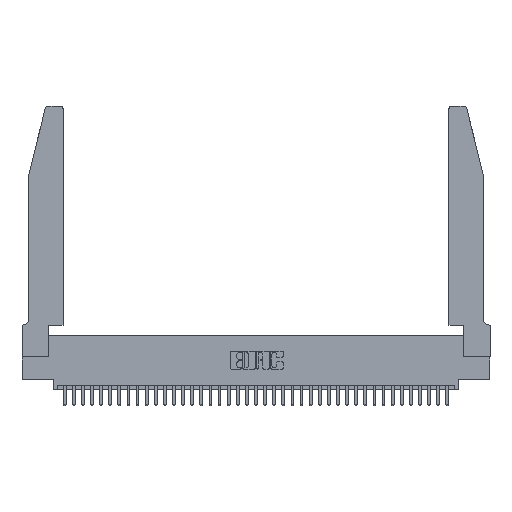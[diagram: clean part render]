
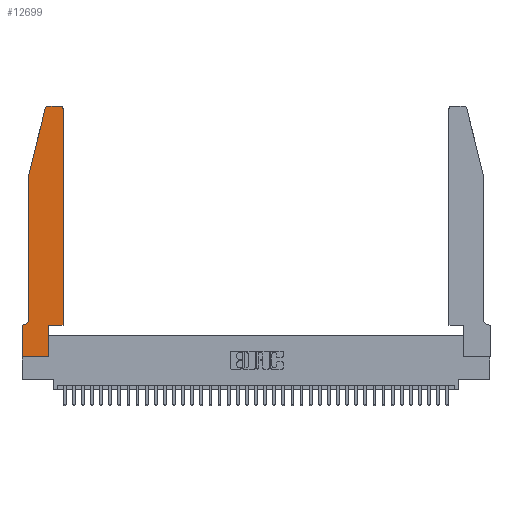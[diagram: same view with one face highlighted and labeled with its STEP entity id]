
A CAD part, top view. The second image highlights one B-rep face of the part: STEP entity #12699.
In plain terms, the highlighted planar face has unit normal (0, 0, 1).
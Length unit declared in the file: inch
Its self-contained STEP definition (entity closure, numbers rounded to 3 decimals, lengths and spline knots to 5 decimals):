
#194 = EDGE_CURVE ( 'NONE', #28728, #16505, #8328, .T. ) ;
#308 = ORIENTED_EDGE ( 'NONE', *, *, #17156, .T. ) ;
#342 = CARTESIAN_POINT ( 'NONE',  ( 0., 0.35, 0.37 ) ) ;
#1009 = EDGE_CURVE ( 'NONE', #16505, #8032, #33854, .T. ) ;
#1348 = CARTESIAN_POINT ( 'NONE',  ( 0.0055, 0.42, 0.37 ) ) ;
#1412 = CARTESIAN_POINT ( 'NONE',  ( 0.4505, 0.35, 0.37 ) ) ;
#1747 = VECTOR ( 'NONE', #4378, 39.37008 ) ;
#2367 = AXIS2_PLACEMENT_3D ( 'NONE', #342, #27251, #9416 ) ;
#2419 = CARTESIAN_POINT ( 'NONE',  ( 0.4505, 0.35, 0.37 ) ) ;
#3085 = VECTOR ( 'NONE', #15691, 39.37008 ) ;
#3551 = AXIS2_PLACEMENT_3D ( 'NONE', #10086, #30923, #13131 ) ;
#3979 = ORIENTED_EDGE ( 'NONE', *, *, #29493, .T. ) ;
#4364 = DIRECTION ( 'NONE',  ( -1., 0., 0. ) ) ;
#4378 = DIRECTION ( 'NONE',  ( 0., -1., 0. ) ) ;
#4823 = VERTEX_POINT ( 'NONE', #13214 ) ;
#4854 = CARTESIAN_POINT ( 'NONE',  ( 0., 0., 0.37 ) ) ;
#5407 = DIRECTION ( 'NONE',  ( 0., 1., 0. ) ) ;
#5885 = FACE_OUTER_BOUND ( 'NONE', #16922, .T. ) ;
#6060 = LINE ( 'NONE', #23362, #22002 ) ;
#6218 = ORIENTED_EDGE ( 'NONE', *, *, #23915, .T. ) ;
#6265 = EDGE_CURVE ( 'NONE', #19348, #28742, #6782, .T. ) ;
#6369 = PLANE ( 'NONE',  #2367 ) ;
#6399 = CARTESIAN_POINT ( 'NONE',  ( 0.0755, 2., 0.37 ) ) ;
#6782 = LINE ( 'NONE', #38151, #37546 ) ;
#7178 = VECTOR ( 'NONE', #22764, 39.37008 ) ;
#7458 = EDGE_CURVE ( 'NONE', #32731, #28728, #30982, .T. ) ;
#7481 = ORIENTED_EDGE ( 'NONE', *, *, #1009, .T. ) ;
#8032 = VERTEX_POINT ( 'NONE', #15784 ) ;
#8328 = LINE ( 'NONE', #30389, #23260 ) ;
#8396 = CARTESIAN_POINT ( 'NONE',  ( 0.0055, 0.35, 0.37 ) ) ;
#8406 = VERTEX_POINT ( 'NONE', #8396 ) ;
#8785 = LINE ( 'NONE', #16609, #1747 ) ;
#9016 = CIRCLE ( 'NONE', #25145, 0.03 ) ;
#9050 = CARTESIAN_POINT ( 'NONE',  ( 0.2865, 0., 0.37 ) ) ;
#9361 = CARTESIAN_POINT ( 'NONE',  ( 0.4205, 2.75, 0.37 ) ) ;
#9416 = DIRECTION ( 'NONE',  ( 1., 0., 0. ) ) ;
#9954 = ORIENTED_EDGE ( 'NONE', *, *, #7458, .T. ) ;
#10081 = CARTESIAN_POINT ( 'NONE',  ( 0.4205, 2.72, 0.37 ) ) ;
#10086 = CARTESIAN_POINT ( 'NONE',  ( 0.284, 2.72, 0.37 ) ) ;
#10368 = ORIENTED_EDGE ( 'NONE', *, *, #22075, .T. ) ;
#11618 = CARTESIAN_POINT ( 'NONE',  ( 0., 0., 0.37 ) ) ;
#12699 = ADVANCED_FACE ( 'NONE', ( #5885 ), #6369, .T. ) ;
#13122 = DIRECTION ( 'NONE',  ( 1., 0., 0. ) ) ;
#13131 = DIRECTION ( 'NONE',  ( 1., 0., 0. ) ) ;
#13214 = CARTESIAN_POINT ( 'NONE',  ( 0.0755, 0.42, 0.37 ) ) ;
#13833 = EDGE_CURVE ( 'NONE', #23992, #32687, #37965, .T. ) ;
#14303 = VECTOR ( 'NONE', #5407, 39.37008 ) ;
#15691 = DIRECTION ( 'NONE',  ( 0., 1., 0. ) ) ;
#15784 = CARTESIAN_POINT ( 'NONE',  ( 0.2865, 0.35, 0.37 ) ) ;
#16247 = CARTESIAN_POINT ( 'NONE',  ( 0.2865, 0.35, 0.37 ) ) ;
#16505 = VERTEX_POINT ( 'NONE', #9050 ) ;
#16609 = CARTESIAN_POINT ( 'NONE',  ( 0.0755, 2., 0.37 ) ) ;
#16922 = EDGE_LOOP ( 'NONE', ( #18839, #31925, #3979, #308, #32676, #20271, #9954, #19948, #7481, #10368, #30151, #6218 ) ) ;
#17156 = EDGE_CURVE ( 'NONE', #34644, #4823, #8785, .T. ) ;
#17176 = CARTESIAN_POINT ( 'NONE',  ( 0.0755, 2., 0.37 ) ) ;
#18839 = ORIENTED_EDGE ( 'NONE', *, *, #6265, .T. ) ;
#19348 = VERTEX_POINT ( 'NONE', #9361 ) ;
#19948 = ORIENTED_EDGE ( 'NONE', *, *, #194, .T. ) ;
#20070 = CIRCLE ( 'NONE', #26383, 0.07 ) ;
#20271 = ORIENTED_EDGE ( 'NONE', *, *, #31197, .T. ) ;
#20625 = CARTESIAN_POINT ( 'NONE',  ( 0.284, 2.75, 0.37 ) ) ;
#21736 = EDGE_CURVE ( 'NONE', #28742, #38479, #32201, .T. ) ;
#21887 = VECTOR ( 'NONE', #36363, 39.37008 ) ;
#22002 = VECTOR ( 'NONE', #29353, 39.37008 ) ;
#22075 = EDGE_CURVE ( 'NONE', #8032, #23992, #6060, .T. ) ;
#22286 = DIRECTION ( 'NONE',  ( 0., 0., -1. ) ) ;
#22313 = CARTESIAN_POINT ( 'NONE',  ( 0.25487, 2.72718, 0.37 ) ) ;
#22764 = DIRECTION ( 'NONE',  ( 0., -1., 0. ) ) ;
#23260 = VECTOR ( 'NONE', #23738, 39.37008 ) ;
#23362 = CARTESIAN_POINT ( 'NONE',  ( 0.4505, 0.35, 0.37 ) ) ;
#23738 = DIRECTION ( 'NONE',  ( 1., 0., 0. ) ) ;
#23915 = EDGE_CURVE ( 'NONE', #32687, #19348, #9016, .T. ) ;
#23992 = VERTEX_POINT ( 'NONE', #1412 ) ;
#24829 = CARTESIAN_POINT ( 'NONE',  ( 0.0755, 0.35, 0.37 ) ) ;
#25145 = AXIS2_PLACEMENT_3D ( 'NONE', #10081, #30919, #13122 ) ;
#25894 = CARTESIAN_POINT ( 'NONE',  ( 0., 0.35, 0.37 ) ) ;
#26383 = AXIS2_PLACEMENT_3D ( 'NONE', #1348, #22286, #4364 ) ;
#27162 = EDGE_CURVE ( 'NONE', #4823, #8406, #20070, .T. ) ;
#27251 = DIRECTION ( 'NONE',  ( 0., 0., 1. ) ) ;
#27813 = DIRECTION ( 'NONE',  ( -1., 0., 0. ) ) ;
#28246 = LINE ( 'NONE', #24829, #35184 ) ;
#28728 = VERTEX_POINT ( 'NONE', #11618 ) ;
#28742 = VERTEX_POINT ( 'NONE', #20625 ) ;
#29353 = DIRECTION ( 'NONE',  ( 1., 0., 0. ) ) ;
#29493 = EDGE_CURVE ( 'NONE', #38479, #34644, #29778, .T. ) ;
#29778 = LINE ( 'NONE', #6399, #21887 ) ;
#30151 = ORIENTED_EDGE ( 'NONE', *, *, #13833, .T. ) ;
#30389 = CARTESIAN_POINT ( 'NONE',  ( 0., 0., 0.37 ) ) ;
#30919 = DIRECTION ( 'NONE',  ( 0., 0., 1. ) ) ;
#30923 = DIRECTION ( 'NONE',  ( 0., 0., 1. ) ) ;
#30982 = LINE ( 'NONE', #4854, #7178 ) ;
#31197 = EDGE_CURVE ( 'NONE', #8406, #32731, #28246, .T. ) ;
#31600 = CARTESIAN_POINT ( 'NONE',  ( 0.4505, 2.72, 0.37 ) ) ;
#31925 = ORIENTED_EDGE ( 'NONE', *, *, #21736, .T. ) ;
#32201 = CIRCLE ( 'NONE', #3551, 0.03 ) ;
#32676 = ORIENTED_EDGE ( 'NONE', *, *, #27162, .T. ) ;
#32687 = VERTEX_POINT ( 'NONE', #31600 ) ;
#32731 = VERTEX_POINT ( 'NONE', #25894 ) ;
#33854 = LINE ( 'NONE', #16247, #3085 ) ;
#34644 = VERTEX_POINT ( 'NONE', #17176 ) ;
#35184 = VECTOR ( 'NONE', #27813, 39.37008 ) ;
#35284 = DIRECTION ( 'NONE',  ( -1., 0., 0. ) ) ;
#36363 = DIRECTION ( 'NONE',  ( -0.239, -0.971, 0. ) ) ;
#37546 = VECTOR ( 'NONE', #35284, 39.37008 ) ;
#37965 = LINE ( 'NONE', #2419, #14303 ) ;
#38151 = CARTESIAN_POINT ( 'NONE',  ( 0.2605, 2.75, 0.37 ) ) ;
#38479 = VERTEX_POINT ( 'NONE', #22313 ) ;
